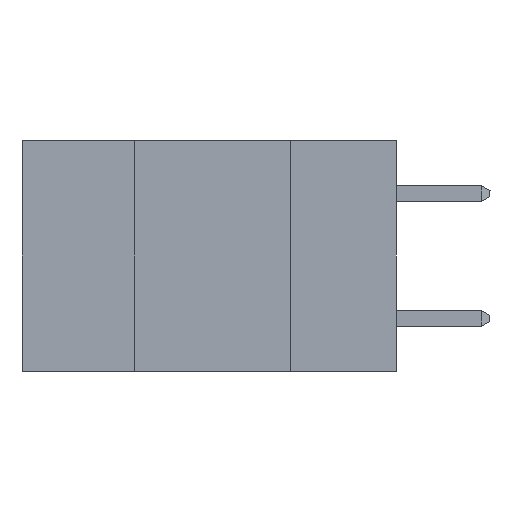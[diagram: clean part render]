
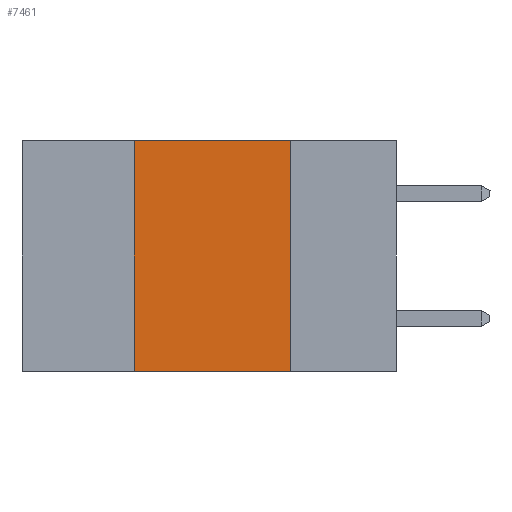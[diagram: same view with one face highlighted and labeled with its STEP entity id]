
A CAD part, left-side view. The second image highlights one B-rep face of the part: STEP entity #7461.
In plain terms, the highlighted planar face has unit normal (-1, 0, 0).
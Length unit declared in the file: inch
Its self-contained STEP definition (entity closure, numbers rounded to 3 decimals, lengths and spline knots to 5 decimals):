
#198 = CARTESIAN_POINT ( 'NONE',  ( 0., 0.6, -0.37 ) ) ;
#393 = LINE ( 'NONE', #10067, #9646 ) ;
#456 = VECTOR ( 'NONE', #4015, 39.37008 ) ;
#622 = CARTESIAN_POINT ( 'NONE',  ( 0., 0.17, -0.37 ) ) ;
#782 = EDGE_CURVE ( 'NONE', #8402, #8156, #7417, .T. ) ;
#1025 = LINE ( 'NONE', #4070, #456 ) ;
#1523 = PLANE ( 'NONE',  #6894 ) ;
#1596 = EDGE_LOOP ( 'NONE', ( #6096, #9181, #6093, #6615 ) ) ;
#2410 = DIRECTION ( 'NONE',  ( 0., 0., -1. ) ) ;
#2506 = CARTESIAN_POINT ( 'NONE',  ( 0., 0.17, 0. ) ) ;
#2742 = CARTESIAN_POINT ( 'NONE',  ( 0., 0.6, 0. ) ) ;
#3067 = EDGE_CURVE ( 'NONE', #8199, #8156, #393, .T. ) ;
#3551 = DIRECTION ( 'NONE',  ( 0., -1., 0. ) ) ;
#3873 = VECTOR ( 'NONE', #8793, 39.37008 ) ;
#4015 = DIRECTION ( 'NONE',  ( 0., 0., 1. ) ) ;
#4070 = CARTESIAN_POINT ( 'NONE',  ( 0., 0.42, 0. ) ) ;
#4313 = VECTOR ( 'NONE', #3551, 39.37008 ) ;
#4452 = CARTESIAN_POINT ( 'NONE',  ( 0., 0.42, 0. ) ) ;
#4582 = CARTESIAN_POINT ( 'NONE',  ( 0., 0.42, -0.37 ) ) ;
#4879 = DIRECTION ( 'NONE',  ( 0., 0., -1. ) ) ;
#4954 = CARTESIAN_POINT ( 'NONE',  ( 0., 0.6, 0. ) ) ;
#5897 = LINE ( 'NONE', #2742, #3873 ) ;
#5958 = FACE_OUTER_BOUND ( 'NONE', #1596, .T. ) ;
#6093 = ORIENTED_EDGE ( 'NONE', *, *, #7114, .F. ) ;
#6096 = ORIENTED_EDGE ( 'NONE', *, *, #3067, .F. ) ;
#6595 = VERTEX_POINT ( 'NONE', #4452 ) ;
#6615 = ORIENTED_EDGE ( 'NONE', *, *, #782, .T. ) ;
#6894 = AXIS2_PLACEMENT_3D ( 'NONE', #4954, #7569, #2410 ) ;
#7114 = EDGE_CURVE ( 'NONE', #8402, #6595, #1025, .T. ) ;
#7417 = LINE ( 'NONE', #198, #4313 ) ;
#7461 = ADVANCED_FACE ( 'NONE', ( #5958 ), #1523, .F. ) ;
#7569 = DIRECTION ( 'NONE',  ( 1., 0., 0. ) ) ;
#8156 = VERTEX_POINT ( 'NONE', #622 ) ;
#8199 = VERTEX_POINT ( 'NONE', #2506 ) ;
#8402 = VERTEX_POINT ( 'NONE', #4582 ) ;
#8793 = DIRECTION ( 'NONE',  ( 0., -1., 0. ) ) ;
#9181 = ORIENTED_EDGE ( 'NONE', *, *, #9605, .F. ) ;
#9605 = EDGE_CURVE ( 'NONE', #6595, #8199, #5897, .T. ) ;
#9646 = VECTOR ( 'NONE', #4879, 39.37008 ) ;
#10067 = CARTESIAN_POINT ( 'NONE',  ( 0., 0.17, 0. ) ) ;
